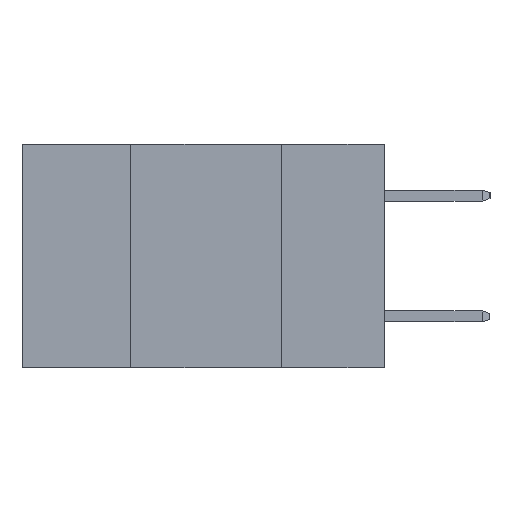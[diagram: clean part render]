
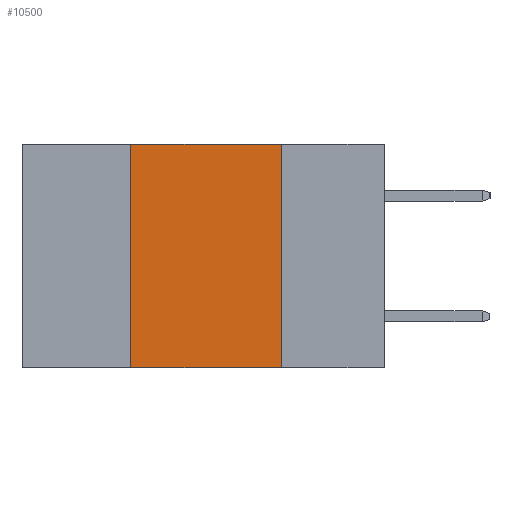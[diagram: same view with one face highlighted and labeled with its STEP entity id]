
A CAD part, left-side view. The second image highlights one B-rep face of the part: STEP entity #10500.
In plain terms, the highlighted planar face has unit normal (-1, 0, 0).
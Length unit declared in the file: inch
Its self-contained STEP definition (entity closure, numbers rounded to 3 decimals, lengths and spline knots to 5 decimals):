
#358 = ORIENTED_EDGE ( 'NONE', *, *, #16654, .F. ) ;
#1512 = CARTESIAN_POINT ( 'NONE',  ( 0., 0.42, 0. ) ) ;
#2388 = LINE ( 'NONE', #4616, #14806 ) ;
#2398 = VERTEX_POINT ( 'NONE', #8589 ) ;
#2710 = ORIENTED_EDGE ( 'NONE', *, *, #10865, .F. ) ;
#2885 = EDGE_CURVE ( 'NONE', #9343, #4308, #6659, .T. ) ;
#3129 = EDGE_LOOP ( 'NONE', ( #5516, #2710, #358, #18737 ) ) ;
#3496 = PLANE ( 'NONE',  #5276 ) ;
#4308 = VERTEX_POINT ( 'NONE', #14893 ) ;
#4423 = FACE_OUTER_BOUND ( 'NONE', #3129, .T. ) ;
#4455 = CARTESIAN_POINT ( 'NONE',  ( 0., 0.17, 0. ) ) ;
#4616 = CARTESIAN_POINT ( 'NONE',  ( 0., 0.6, 0. ) ) ;
#4907 = DIRECTION ( 'NONE',  ( 0., 0., 1. ) ) ;
#5110 = DIRECTION ( 'NONE',  ( 0., 0., -1. ) ) ;
#5276 = AXIS2_PLACEMENT_3D ( 'NONE', #8349, #14801, #5110 ) ;
#5516 = ORIENTED_EDGE ( 'NONE', *, *, #12317, .F. ) ;
#6659 = LINE ( 'NONE', #13591, #9940 ) ;
#7439 = VECTOR ( 'NONE', #20737, 39.37008 ) ;
#8349 = CARTESIAN_POINT ( 'NONE',  ( 0., 0.6, 0. ) ) ;
#8589 = CARTESIAN_POINT ( 'NONE',  ( 0., 0.42, 0. ) ) ;
#9267 = VERTEX_POINT ( 'NONE', #18349 ) ;
#9343 = VERTEX_POINT ( 'NONE', #10521 ) ;
#9940 = VECTOR ( 'NONE', #14033, 39.37008 ) ;
#10500 = ADVANCED_FACE ( 'NONE', ( #4423 ), #3496, .F. ) ;
#10521 = CARTESIAN_POINT ( 'NONE',  ( 0., 0.42, -0.37 ) ) ;
#10865 = EDGE_CURVE ( 'NONE', #2398, #9267, #2388, .T. ) ;
#11778 = LINE ( 'NONE', #4455, #7439 ) ;
#12317 = EDGE_CURVE ( 'NONE', #9267, #4308, #11778, .T. ) ;
#13176 = VECTOR ( 'NONE', #4907, 39.37008 ) ;
#13591 = CARTESIAN_POINT ( 'NONE',  ( 0., 0.6, -0.37 ) ) ;
#14033 = DIRECTION ( 'NONE',  ( 0., -1., 0. ) ) ;
#14801 = DIRECTION ( 'NONE',  ( 1., 0., 0. ) ) ;
#14806 = VECTOR ( 'NONE', #17590, 39.37008 ) ;
#14893 = CARTESIAN_POINT ( 'NONE',  ( 0., 0.17, -0.37 ) ) ;
#16654 = EDGE_CURVE ( 'NONE', #9343, #2398, #17461, .T. ) ;
#17461 = LINE ( 'NONE', #1512, #13176 ) ;
#17590 = DIRECTION ( 'NONE',  ( 0., -1., 0. ) ) ;
#18349 = CARTESIAN_POINT ( 'NONE',  ( 0., 0.17, 0. ) ) ;
#18737 = ORIENTED_EDGE ( 'NONE', *, *, #2885, .T. ) ;
#20737 = DIRECTION ( 'NONE',  ( 0., 0., -1. ) ) ;
